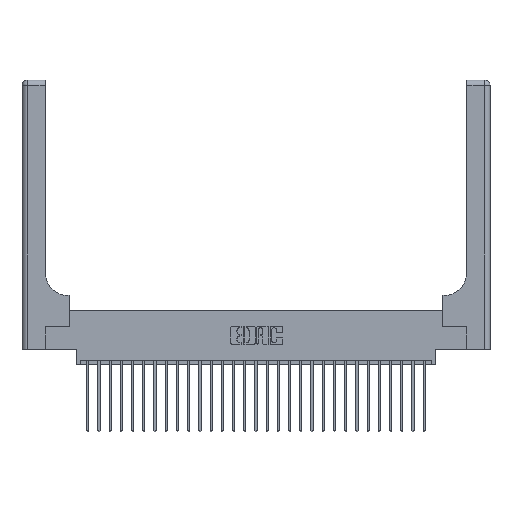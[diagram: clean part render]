
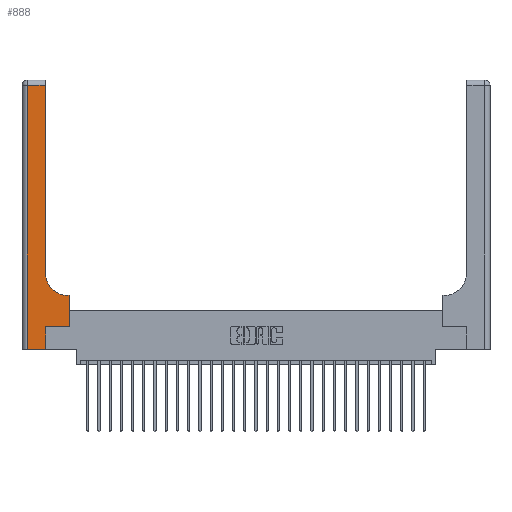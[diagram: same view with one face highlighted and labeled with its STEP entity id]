
A CAD part, top view. The second image highlights one B-rep face of the part: STEP entity #888.
In plain terms, the highlighted planar face has unit normal (0, 0, 1).
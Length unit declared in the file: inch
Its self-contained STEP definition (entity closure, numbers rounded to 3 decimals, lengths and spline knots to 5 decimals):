
#153 = VERTEX_POINT ( 'NONE', #22901 ) ;
#304 = ORIENTED_EDGE ( 'NONE', *, *, #1890, .T. ) ;
#462 = EDGE_CURVE ( 'NONE', #13043, #24673, #5542, .T. ) ;
#888 = ADVANCED_FACE ( 'NONE', ( #1240 ), #26783, .F. ) ;
#1072 = DIRECTION ( 'NONE',  ( 1., 0., 0. ) ) ;
#1105 = CARTESIAN_POINT ( 'NONE',  ( 0.06, 3., 0.37 ) ) ;
#1163 = DIRECTION ( 'NONE',  ( 0., -1., 0. ) ) ;
#1240 = FACE_OUTER_BOUND ( 'NONE', #10404, .T. ) ;
#1340 = CARTESIAN_POINT ( 'NONE',  ( 0., 0., 0.37 ) ) ;
#1574 = CARTESIAN_POINT ( 'NONE',  ( 0.265, 0., 0.37 ) ) ;
#1767 = DIRECTION ( 'NONE',  ( -1., 0., 0. ) ) ;
#1886 = CARTESIAN_POINT ( 'NONE',  ( 0.51, 0.6, 0.37 ) ) ;
#1890 = EDGE_CURVE ( 'NONE', #25692, #13043, #12190, .T. ) ;
#2164 = VERTEX_POINT ( 'NONE', #5379 ) ;
#2291 = ORIENTED_EDGE ( 'NONE', *, *, #21048, .T. ) ;
#3072 = LINE ( 'NONE', #1340, #13518 ) ;
#3472 = DIRECTION ( 'NONE',  ( 1., 0., 0. ) ) ;
#3660 = DIRECTION ( 'NONE',  ( 0., 0., -1. ) ) ;
#3968 = LINE ( 'NONE', #20348, #24917 ) ;
#4533 = EDGE_CURVE ( 'NONE', #2164, #153, #17727, .T. ) ;
#5031 = DIRECTION ( 'NONE',  ( 0., 1., 0. ) ) ;
#5379 = CARTESIAN_POINT ( 'NONE',  ( 0.528, 0.25, 0.37 ) ) ;
#5542 = LINE ( 'NONE', #1105, #16031 ) ;
#6342 = LINE ( 'NONE', #13199, #11892 ) ;
#6458 = CARTESIAN_POINT ( 'NONE',  ( 0.26, 2.94, 0.37 ) ) ;
#6555 = ORIENTED_EDGE ( 'NONE', *, *, #462, .T. ) ;
#8857 = CARTESIAN_POINT ( 'NONE',  ( 0., 2.94, 0.37 ) ) ;
#9169 = ORIENTED_EDGE ( 'NONE', *, *, #4533, .T. ) ;
#9257 = EDGE_CURVE ( 'NONE', #24673, #15988, #3072, .T. ) ;
#9822 = ORIENTED_EDGE ( 'NONE', *, *, #24852, .T. ) ;
#10404 = EDGE_LOOP ( 'NONE', ( #16382, #304, #6555, #17733, #2291, #24571, #9169, #25850, #9822 ) ) ;
#10405 = EDGE_CURVE ( 'NONE', #23471, #2164, #3968, .T. ) ;
#11447 = VECTOR ( 'NONE', #16030, 39.37008 ) ;
#11892 = VECTOR ( 'NONE', #25709, 39.37008 ) ;
#12190 = LINE ( 'NONE', #8857, #17822 ) ;
#12673 = VECTOR ( 'NONE', #21226, 39.37008 ) ;
#13043 = VERTEX_POINT ( 'NONE', #26234 ) ;
#13199 = CARTESIAN_POINT ( 'NONE',  ( 0.26, 3., 0.37 ) ) ;
#13518 = VECTOR ( 'NONE', #3472, 39.37008 ) ;
#13728 = LINE ( 'NONE', #21793, #19345 ) ;
#13807 = CIRCLE ( 'NONE', #21847, 0.25 ) ;
#13950 = CARTESIAN_POINT ( 'NONE',  ( 0.265, 0.25, 0.37 ) ) ;
#14302 = DIRECTION ( 'NONE',  ( 0., 0., -1. ) ) ;
#15376 = VERTEX_POINT ( 'NONE', #1886 ) ;
#15498 = EDGE_CURVE ( 'NONE', #153, #15376, #18269, .T. ) ;
#15587 = CARTESIAN_POINT ( 'NONE',  ( 0.06, 0., 0.37 ) ) ;
#15988 = VERTEX_POINT ( 'NONE', #1574 ) ;
#16030 = DIRECTION ( 'NONE',  ( 0., 1., 0. ) ) ;
#16031 = VECTOR ( 'NONE', #1163, 39.37008 ) ;
#16207 = CARTESIAN_POINT ( 'NONE',  ( 0.51, 0.85, 0.37 ) ) ;
#16382 = ORIENTED_EDGE ( 'NONE', *, *, #18227, .T. ) ;
#17112 = CARTESIAN_POINT ( 'NONE',  ( 0.26, 0.85, 0.37 ) ) ;
#17727 = LINE ( 'NONE', #22429, #11447 ) ;
#17733 = ORIENTED_EDGE ( 'NONE', *, *, #9257, .T. ) ;
#17822 = VECTOR ( 'NONE', #23514, 39.37008 ) ;
#18227 = EDGE_CURVE ( 'NONE', #26895, #25692, #6342, .T. ) ;
#18269 = LINE ( 'NONE', #25112, #12673 ) ;
#18323 = DIRECTION ( 'NONE',  ( 1., 0., 0. ) ) ;
#19345 = VECTOR ( 'NONE', #5031, 39.37008 ) ;
#20348 = CARTESIAN_POINT ( 'NONE',  ( 0.265, 0.25, 0.37 ) ) ;
#21048 = EDGE_CURVE ( 'NONE', #15988, #23471, #13728, .T. ) ;
#21149 = AXIS2_PLACEMENT_3D ( 'NONE', #22657, #14302, #1767 ) ;
#21226 = DIRECTION ( 'NONE',  ( -1., 0., 0. ) ) ;
#21793 = CARTESIAN_POINT ( 'NONE',  ( 0.265, 0., 0.37 ) ) ;
#21847 = AXIS2_PLACEMENT_3D ( 'NONE', #16207, #3660, #18323 ) ;
#22429 = CARTESIAN_POINT ( 'NONE',  ( 0.528, 0.25, 0.37 ) ) ;
#22657 = CARTESIAN_POINT ( 'NONE',  ( 0., 3., 0.37 ) ) ;
#22901 = CARTESIAN_POINT ( 'NONE',  ( 0.528, 0.6, 0.37 ) ) ;
#23471 = VERTEX_POINT ( 'NONE', #13950 ) ;
#23514 = DIRECTION ( 'NONE',  ( -1., 0., 0. ) ) ;
#24571 = ORIENTED_EDGE ( 'NONE', *, *, #10405, .T. ) ;
#24673 = VERTEX_POINT ( 'NONE', #15587 ) ;
#24852 = EDGE_CURVE ( 'NONE', #15376, #26895, #13807, .T. ) ;
#24917 = VECTOR ( 'NONE', #1072, 39.37008 ) ;
#25112 = CARTESIAN_POINT ( 'NONE',  ( 0.26, 0.6, 0.37 ) ) ;
#25692 = VERTEX_POINT ( 'NONE', #6458 ) ;
#25709 = DIRECTION ( 'NONE',  ( 0., 1., 0. ) ) ;
#25850 = ORIENTED_EDGE ( 'NONE', *, *, #15498, .T. ) ;
#26234 = CARTESIAN_POINT ( 'NONE',  ( 0.06, 2.94, 0.37 ) ) ;
#26783 = PLANE ( 'NONE',  #21149 ) ;
#26895 = VERTEX_POINT ( 'NONE', #17112 ) ;
